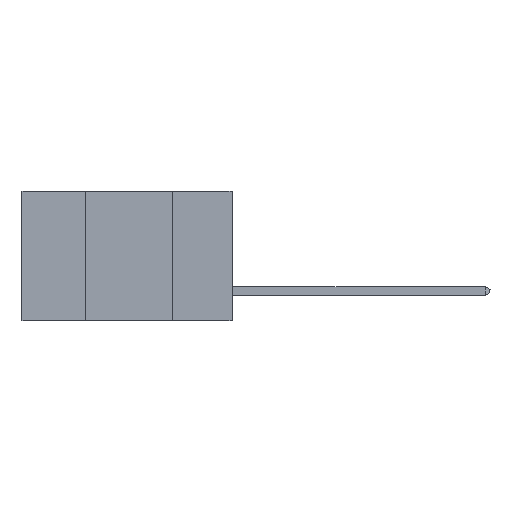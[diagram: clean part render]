
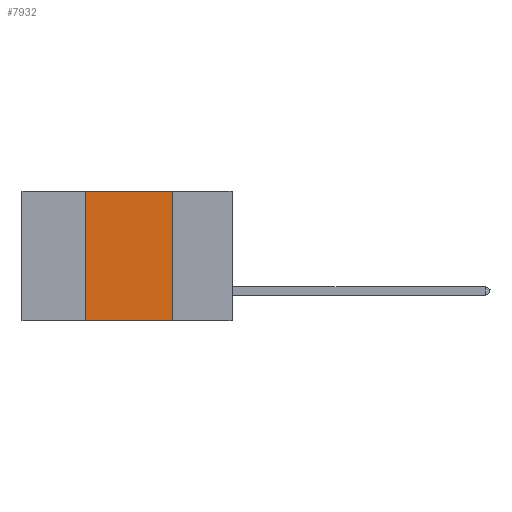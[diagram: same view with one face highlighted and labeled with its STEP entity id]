
A CAD part, left-side view. The second image highlights one B-rep face of the part: STEP entity #7932.
In plain terms, the highlighted planar face has unit normal (-1, 0, 0).
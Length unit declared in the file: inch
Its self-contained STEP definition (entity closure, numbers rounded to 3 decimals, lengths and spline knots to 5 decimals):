
#123 = EDGE_CURVE ( 'NONE', #17034, #11452, #6539, .T. ) ;
#514 = CARTESIAN_POINT ( 'NONE',  ( 0., 0.42, -0.37 ) ) ;
#1197 = VECTOR ( 'NONE', #6592, 39.37008 ) ;
#2103 = ORIENTED_EDGE ( 'NONE', *, *, #123, .F. ) ;
#3896 = LINE ( 'NONE', #20254, #20411 ) ;
#4396 = DIRECTION ( 'NONE',  ( 0., 0., -1. ) ) ;
#4661 = CARTESIAN_POINT ( 'NONE',  ( 0., 0.42, 0. ) ) ;
#5607 = LINE ( 'NONE', #6635, #12227 ) ;
#6539 = LINE ( 'NONE', #7484, #14380 ) ;
#6592 = DIRECTION ( 'NONE',  ( 0., 0., 1. ) ) ;
#6635 = CARTESIAN_POINT ( 'NONE',  ( 0., 0.6, -0.37 ) ) ;
#7484 = CARTESIAN_POINT ( 'NONE',  ( 0., 0.17, 0. ) ) ;
#7932 = ADVANCED_FACE ( 'NONE', ( #16071 ), #21377, .F. ) ;
#11452 = VERTEX_POINT ( 'NONE', #17069 ) ;
#11651 = EDGE_CURVE ( 'NONE', #15310, #13432, #14111, .T. ) ;
#12227 = VECTOR ( 'NONE', #16286, 39.37008 ) ;
#12235 = CARTESIAN_POINT ( 'NONE',  ( 0., 0.6, 0. ) ) ;
#13432 = VERTEX_POINT ( 'NONE', #4661 ) ;
#14111 = LINE ( 'NONE', #21816, #1197 ) ;
#14380 = VECTOR ( 'NONE', #24520, 39.37008 ) ;
#14970 = EDGE_CURVE ( 'NONE', #15310, #11452, #5607, .T. ) ;
#15310 = VERTEX_POINT ( 'NONE', #514 ) ;
#15705 = CARTESIAN_POINT ( 'NONE',  ( 0., 0.17, 0. ) ) ;
#16071 = FACE_OUTER_BOUND ( 'NONE', #18348, .T. ) ;
#16286 = DIRECTION ( 'NONE',  ( 0., -1., 0. ) ) ;
#16348 = ORIENTED_EDGE ( 'NONE', *, *, #11651, .F. ) ;
#17034 = VERTEX_POINT ( 'NONE', #15705 ) ;
#17069 = CARTESIAN_POINT ( 'NONE',  ( 0., 0.17, -0.37 ) ) ;
#17444 = ORIENTED_EDGE ( 'NONE', *, *, #14970, .T. ) ;
#17925 = AXIS2_PLACEMENT_3D ( 'NONE', #12235, #19555, #4396 ) ;
#18348 = EDGE_LOOP ( 'NONE', ( #2103, #22753, #16348, #17444 ) ) ;
#19555 = DIRECTION ( 'NONE',  ( 1., 0., 0. ) ) ;
#20254 = CARTESIAN_POINT ( 'NONE',  ( 0., 0.6, 0. ) ) ;
#20411 = VECTOR ( 'NONE', #22164, 39.37008 ) ;
#21377 = PLANE ( 'NONE',  #17925 ) ;
#21816 = CARTESIAN_POINT ( 'NONE',  ( 0., 0.42, 0. ) ) ;
#22164 = DIRECTION ( 'NONE',  ( 0., -1., 0. ) ) ;
#22753 = ORIENTED_EDGE ( 'NONE', *, *, #23850, .F. ) ;
#23850 = EDGE_CURVE ( 'NONE', #13432, #17034, #3896, .T. ) ;
#24520 = DIRECTION ( 'NONE',  ( 0., 0., -1. ) ) ;
